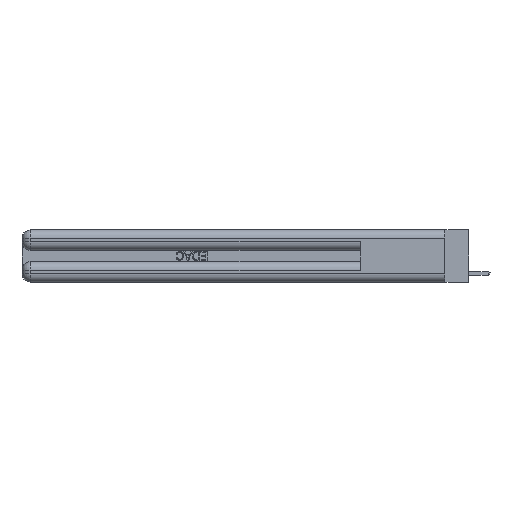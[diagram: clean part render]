
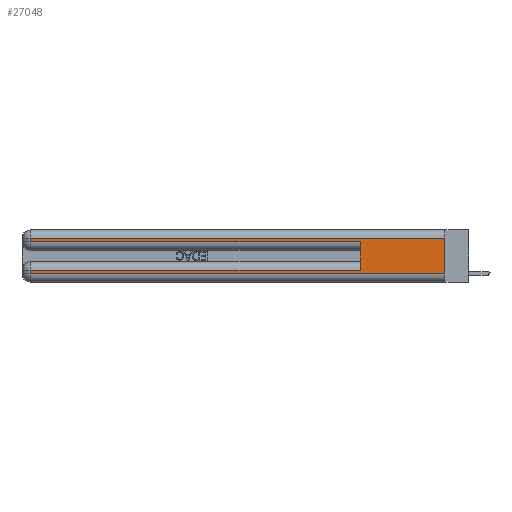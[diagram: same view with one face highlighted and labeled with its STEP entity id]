
A CAD part, left-side view. The second image highlights one B-rep face of the part: STEP entity #27048.
In plain terms, the highlighted planar face has unit normal (-1, 0, 0).
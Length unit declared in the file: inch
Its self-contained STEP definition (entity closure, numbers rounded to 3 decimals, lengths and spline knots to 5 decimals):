
#39 = CARTESIAN_POINT ( 'NONE',  ( 0., 2.94, 0.06 ) ) ;
#1227 = ORIENTED_EDGE ( 'NONE', *, *, #28492, .T. ) ;
#1229 = VERTEX_POINT ( 'NONE', #6356 ) ;
#2094 = CARTESIAN_POINT ( 'NONE',  ( 0., 0., 0.06 ) ) ;
#2318 = VECTOR ( 'NONE', #18583, 39.37008 ) ;
#3095 = DIRECTION ( 'NONE',  ( 0., 1., 0. ) ) ;
#3348 = EDGE_CURVE ( 'NONE', #15028, #25999, #17248, .T. ) ;
#4205 = VECTOR ( 'NONE', #5331, 39.37008 ) ;
#4224 = CARTESIAN_POINT ( 'NONE',  ( 0., 2.94, 0.285 ) ) ;
#4250 = VERTEX_POINT ( 'NONE', #4298 ) ;
#4298 = CARTESIAN_POINT ( 'NONE',  ( 0., 0.6, 0.285 ) ) ;
#4706 = DIRECTION ( 'NONE',  ( 0., 0., -1. ) ) ;
#4759 = CARTESIAN_POINT ( 'NONE',  ( 0., 0., 0.31 ) ) ;
#4819 = CARTESIAN_POINT ( 'NONE',  ( 0., 0.6, 0.145 ) ) ;
#5331 = DIRECTION ( 'NONE',  ( 0., 0., 1. ) ) ;
#5800 = ORIENTED_EDGE ( 'NONE', *, *, #18001, .T. ) ;
#6273 = LINE ( 'NONE', #22982, #18229 ) ;
#6356 = CARTESIAN_POINT ( 'NONE',  ( 0., 0.6, 0.085 ) ) ;
#6468 = CARTESIAN_POINT ( 'NONE',  ( 0., 2.94, 0.37 ) ) ;
#6528 = EDGE_CURVE ( 'NONE', #21302, #14237, #18329, .T. ) ;
#8869 = LINE ( 'NONE', #18330, #26755 ) ;
#9106 = PLANE ( 'NONE',  #25520 ) ;
#11387 = DIRECTION ( 'NONE',  ( 0., 0., -1. ) ) ;
#11432 = DIRECTION ( 'NONE',  ( 0., 1., 0. ) ) ;
#11488 = CARTESIAN_POINT ( 'NONE',  ( 0., 0., 0.37 ) ) ;
#11531 = CARTESIAN_POINT ( 'NONE',  ( 0., 0., 0.37 ) ) ;
#11630 = DIRECTION ( 'NONE',  ( 0., 0., -1. ) ) ;
#11804 = LINE ( 'NONE', #6468, #27826 ) ;
#11896 = VERTEX_POINT ( 'NONE', #4224 ) ;
#13260 = EDGE_CURVE ( 'NONE', #1229, #4250, #19915, .T. ) ;
#14023 = CARTESIAN_POINT ( 'NONE',  ( 0., 2.94, 0.37 ) ) ;
#14146 = LINE ( 'NONE', #22480, #14503 ) ;
#14237 = VERTEX_POINT ( 'NONE', #39 ) ;
#14503 = VECTOR ( 'NONE', #29692, 39.37008 ) ;
#14995 = ORIENTED_EDGE ( 'NONE', *, *, #28673, .T. ) ;
#15028 = VERTEX_POINT ( 'NONE', #19784 ) ;
#15313 = VECTOR ( 'NONE', #3095, 39.37008 ) ;
#15437 = DIRECTION ( 'NONE',  ( 0., -1., 0. ) ) ;
#17248 = LINE ( 'NONE', #11488, #2318 ) ;
#17377 = ORIENTED_EDGE ( 'NONE', *, *, #13260, .F. ) ;
#18001 = EDGE_CURVE ( 'NONE', #24065, #11896, #11804, .T. ) ;
#18229 = VECTOR ( 'NONE', #15437, 39.37008 ) ;
#18329 = LINE ( 'NONE', #14023, #19807 ) ;
#18330 = CARTESIAN_POINT ( 'NONE',  ( 0., 0., 0.085 ) ) ;
#18583 = DIRECTION ( 'NONE',  ( 0., 0., -1. ) ) ;
#19784 = CARTESIAN_POINT ( 'NONE',  ( 0., 0., 0.31 ) ) ;
#19807 = VECTOR ( 'NONE', #4706, 39.37008 ) ;
#19813 = ORIENTED_EDGE ( 'NONE', *, *, #3348, .F. ) ;
#19915 = LINE ( 'NONE', #4819, #4205 ) ;
#20487 = LINE ( 'NONE', #4759, #15313 ) ;
#20914 = CARTESIAN_POINT ( 'NONE',  ( 0., 2.94, 0.085 ) ) ;
#21302 = VERTEX_POINT ( 'NONE', #20914 ) ;
#22480 = CARTESIAN_POINT ( 'NONE',  ( 0., 0., 0.285 ) ) ;
#22518 = CARTESIAN_POINT ( 'NONE',  ( 0., 2.94, 0.31 ) ) ;
#22982 = CARTESIAN_POINT ( 'NONE',  ( 0., 0., 0.06 ) ) ;
#23271 = DIRECTION ( 'NONE',  ( 1., 0., 0. ) ) ;
#23508 = FACE_OUTER_BOUND ( 'NONE', #29804, .T. ) ;
#23748 = ORIENTED_EDGE ( 'NONE', *, *, #30456, .T. ) ;
#24065 = VERTEX_POINT ( 'NONE', #22518 ) ;
#25150 = ORIENTED_EDGE ( 'NONE', *, *, #6528, .T. ) ;
#25520 = AXIS2_PLACEMENT_3D ( 'NONE', #11531, #23271, #11630 ) ;
#25999 = VERTEX_POINT ( 'NONE', #2094 ) ;
#26755 = VECTOR ( 'NONE', #11432, 39.37008 ) ;
#27048 = ADVANCED_FACE ( 'NONE', ( #23508 ), #9106, .F. ) ;
#27826 = VECTOR ( 'NONE', #11387, 39.37008 ) ;
#28492 = EDGE_CURVE ( 'NONE', #11896, #4250, #14146, .T. ) ;
#28596 = EDGE_CURVE ( 'NONE', #14237, #25999, #6273, .T. ) ;
#28673 = EDGE_CURVE ( 'NONE', #1229, #21302, #8869, .T. ) ;
#29505 = ORIENTED_EDGE ( 'NONE', *, *, #28596, .T. ) ;
#29692 = DIRECTION ( 'NONE',  ( 0., -1., 0. ) ) ;
#29804 = EDGE_LOOP ( 'NONE', ( #19813, #23748, #5800, #1227, #17377, #14995, #25150, #29505 ) ) ;
#30456 = EDGE_CURVE ( 'NONE', #15028, #24065, #20487, .T. ) ;
